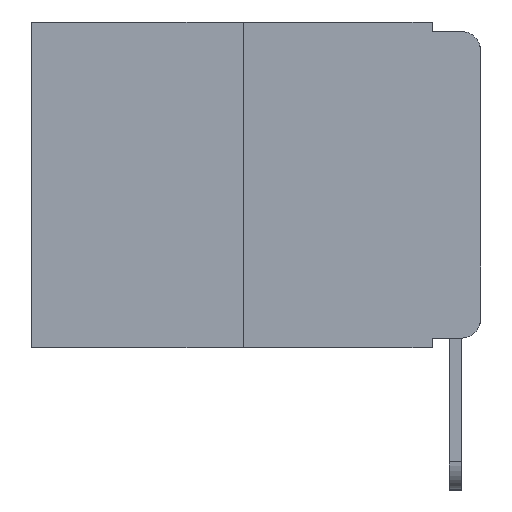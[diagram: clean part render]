
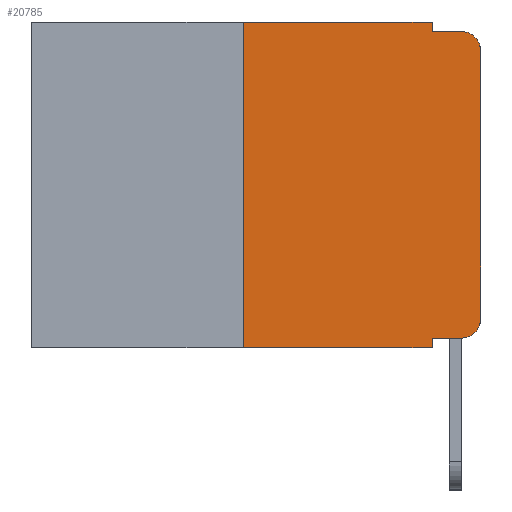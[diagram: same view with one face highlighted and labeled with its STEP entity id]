
A CAD part, left-side view. The second image highlights one B-rep face of the part: STEP entity #20785.
In plain terms, the highlighted planar face has unit normal (-1, 0, 0).
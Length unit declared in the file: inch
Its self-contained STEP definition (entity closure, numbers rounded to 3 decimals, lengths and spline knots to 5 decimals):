
#666 = DIRECTION ( 'NONE',  ( -1., 0., 0. ) ) ;
#696 = DIRECTION ( 'NONE',  ( 0., -1., 0. ) ) ;
#841 = CARTESIAN_POINT ( 'NONE',  ( 0., 0.02, -0.01 ) ) ;
#1135 = EDGE_CURVE ( 'NONE', #3943, #17567, #7066, .T. ) ;
#1288 = FACE_OUTER_BOUND ( 'NONE', #8490, .T. ) ;
#1350 = CARTESIAN_POINT ( 'NONE',  ( 0., 0.02, -0.333 ) ) ;
#1468 = CARTESIAN_POINT ( 'NONE',  ( 0., 0.051, 0. ) ) ;
#1623 = AXIS2_PLACEMENT_3D ( 'NONE', #7142, #11776, #12185 ) ;
#1992 = LINE ( 'NONE', #12277, #7147 ) ;
#2546 = CARTESIAN_POINT ( 'NONE',  ( 0., 0., 0. ) ) ;
#3457 = LINE ( 'NONE', #15611, #5017 ) ;
#3712 = VERTEX_POINT ( 'NONE', #9119 ) ;
#3748 = LINE ( 'NONE', #9280, #11248 ) ;
#3933 = DIRECTION ( 'NONE',  ( 0., 0., -1. ) ) ;
#3943 = VERTEX_POINT ( 'NONE', #1350 ) ;
#4274 = EDGE_CURVE ( 'NONE', #3712, #11915, #19372, .T. ) ;
#5017 = VECTOR ( 'NONE', #17271, 39.37008 ) ;
#5110 = VERTEX_POINT ( 'NONE', #16075 ) ;
#5330 = CARTESIAN_POINT ( 'NONE',  ( 0., 0.051, -0.333 ) ) ;
#5442 = ORIENTED_EDGE ( 'NONE', *, *, #20965, .F. ) ;
#5903 = EDGE_CURVE ( 'NONE', #9024, #15075, #20016, .T. ) ;
#6229 = DIRECTION ( 'NONE',  ( 0., 0., 1. ) ) ;
#6234 = ORIENTED_EDGE ( 'NONE', *, *, #6681, .F. ) ;
#6431 = ORIENTED_EDGE ( 'NONE', *, *, #1135, .T. ) ;
#6681 = EDGE_CURVE ( 'NONE', #18193, #11701, #17125, .T. ) ;
#7066 = CIRCLE ( 'NONE', #7232, 0.02 ) ;
#7142 = CARTESIAN_POINT ( 'NONE',  ( 0., 0.02, -0.03 ) ) ;
#7147 = VECTOR ( 'NONE', #13773, 39.37008 ) ;
#7187 = CARTESIAN_POINT ( 'NONE',  ( 0., 0.02, -0.313 ) ) ;
#7232 = AXIS2_PLACEMENT_3D ( 'NONE', #7187, #666, #3933 ) ;
#7655 = CARTESIAN_POINT ( 'NONE',  ( 0., 0.473, 0. ) ) ;
#7782 = CARTESIAN_POINT ( 'NONE',  ( 0., 0.051, -0.01 ) ) ;
#8490 = EDGE_LOOP ( 'NONE', ( #10269, #16146, #6234, #10368, #10547, #19756, #10385, #5442, #17610, #6431 ) ) ;
#8822 = CARTESIAN_POINT ( 'NONE',  ( 0., 0.051, -0.343 ) ) ;
#8847 = VECTOR ( 'NONE', #20654, 39.37008 ) ;
#8863 = LINE ( 'NONE', #2546, #17324 ) ;
#9024 = VERTEX_POINT ( 'NONE', #12177 ) ;
#9119 = CARTESIAN_POINT ( 'NONE',  ( 0., 0.25, 0. ) ) ;
#9280 = CARTESIAN_POINT ( 'NONE',  ( 0., 0.051, -0.333 ) ) ;
#9545 = DIRECTION ( 'NONE',  ( 0., 0., -1. ) ) ;
#9864 = DIRECTION ( 'NONE',  ( 0., -1., 0. ) ) ;
#10027 = EDGE_CURVE ( 'NONE', #12330, #3943, #3748, .T. ) ;
#10269 = ORIENTED_EDGE ( 'NONE', *, *, #14598, .T. ) ;
#10368 = ORIENTED_EDGE ( 'NONE', *, *, #11732, .F. ) ;
#10385 = ORIENTED_EDGE ( 'NONE', *, *, #5903, .T. ) ;
#10547 = ORIENTED_EDGE ( 'NONE', *, *, #4274, .F. ) ;
#11232 = VECTOR ( 'NONE', #696, 39.37008 ) ;
#11248 = VECTOR ( 'NONE', #19214, 39.37008 ) ;
#11701 = VERTEX_POINT ( 'NONE', #841 ) ;
#11732 = EDGE_CURVE ( 'NONE', #11915, #18193, #1992, .T. ) ;
#11776 = DIRECTION ( 'NONE',  ( -1., 0., 0. ) ) ;
#11915 = VERTEX_POINT ( 'NONE', #20819 ) ;
#12177 = CARTESIAN_POINT ( 'NONE',  ( 0., 0.25, -0.343 ) ) ;
#12185 = DIRECTION ( 'NONE',  ( 0., 0., -1. ) ) ;
#12277 = CARTESIAN_POINT ( 'NONE',  ( 0., 0.051, 0. ) ) ;
#12330 = VERTEX_POINT ( 'NONE', #5330 ) ;
#12633 = DIRECTION ( 'NONE',  ( 0., 0., -1. ) ) ;
#13634 = CARTESIAN_POINT ( 'NONE',  ( 0., 0.051, -0.01 ) ) ;
#13773 = DIRECTION ( 'NONE',  ( 0., 0., -1. ) ) ;
#14481 = CIRCLE ( 'NONE', #1623, 0.02 ) ;
#14598 = EDGE_CURVE ( 'NONE', #17567, #5110, #8863, .T. ) ;
#15031 = EDGE_CURVE ( 'NONE', #5110, #11701, #14481, .T. ) ;
#15075 = VERTEX_POINT ( 'NONE', #8822 ) ;
#15611 = CARTESIAN_POINT ( 'NONE',  ( 0., 0.25, 0. ) ) ;
#15663 = CARTESIAN_POINT ( 'NONE',  ( 0., 0.473, 0. ) ) ;
#16075 = CARTESIAN_POINT ( 'NONE',  ( 0., 0., -0.03 ) ) ;
#16146 = ORIENTED_EDGE ( 'NONE', *, *, #15031, .T. ) ;
#16683 = LINE ( 'NONE', #1468, #20540 ) ;
#17125 = LINE ( 'NONE', #13634, #11232 ) ;
#17271 = DIRECTION ( 'NONE',  ( 0., 0., 1. ) ) ;
#17324 = VECTOR ( 'NONE', #6229, 39.37008 ) ;
#17407 = DIRECTION ( 'NONE',  ( 1., 0., 0. ) ) ;
#17438 = EDGE_CURVE ( 'NONE', #9024, #3712, #3457, .T. ) ;
#17567 = VERTEX_POINT ( 'NONE', #21037 ) ;
#17610 = ORIENTED_EDGE ( 'NONE', *, *, #10027, .T. ) ;
#18155 = AXIS2_PLACEMENT_3D ( 'NONE', #7655, #17407, #12633 ) ;
#18193 = VERTEX_POINT ( 'NONE', #7782 ) ;
#19214 = DIRECTION ( 'NONE',  ( 0., -1., 0. ) ) ;
#19372 = LINE ( 'NONE', #15663, #8847 ) ;
#19383 = CARTESIAN_POINT ( 'NONE',  ( 0., 0.473, -0.343 ) ) ;
#19756 = ORIENTED_EDGE ( 'NONE', *, *, #17438, .F. ) ;
#20016 = LINE ( 'NONE', #19383, #21053 ) ;
#20540 = VECTOR ( 'NONE', #9545, 39.37008 ) ;
#20654 = DIRECTION ( 'NONE',  ( 0., -1., 0. ) ) ;
#20734 = PLANE ( 'NONE',  #18155 ) ;
#20785 = ADVANCED_FACE ( 'NONE', ( #1288 ), #20734, .F. ) ;
#20819 = CARTESIAN_POINT ( 'NONE',  ( 0., 0.051, 0. ) ) ;
#20965 = EDGE_CURVE ( 'NONE', #12330, #15075, #16683, .T. ) ;
#21037 = CARTESIAN_POINT ( 'NONE',  ( 0., 0., -0.313 ) ) ;
#21053 = VECTOR ( 'NONE', #9864, 39.37008 ) ;
